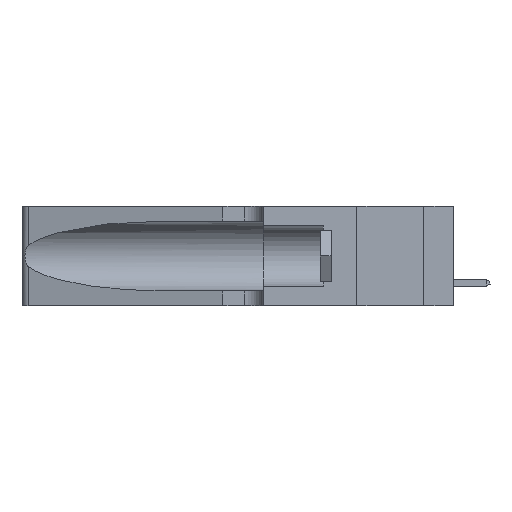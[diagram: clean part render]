
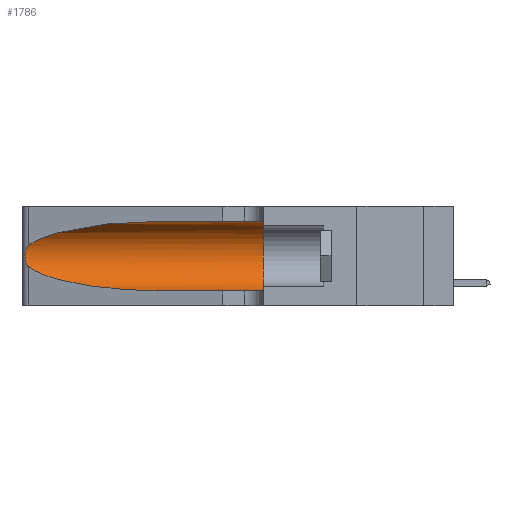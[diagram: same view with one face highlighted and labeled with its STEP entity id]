
A CAD part, left-side view. The second image highlights one B-rep face of the part: STEP entity #1786.
In plain terms, the highlighted cylindrical face has radius 3.308 mm (diameter 6.617 mm), a partial arc.
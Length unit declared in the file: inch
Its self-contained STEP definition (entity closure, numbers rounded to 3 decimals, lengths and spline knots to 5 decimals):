
#256 = FACE_OUTER_BOUND ( 'NONE', #6299, .T. ) ;
#331 = VERTEX_POINT ( 'NONE', #4029 ) ;
#347 = DIRECTION ( 'NONE',  ( 0., -1., 0. ) ) ;
#350 = VERTEX_POINT ( 'NONE', #19721 ) ;
#406 = VERTEX_POINT ( 'NONE', #17845 ) ;
#582 = DIRECTION ( 'NONE',  ( 0., 1., 0. ) ) ;
#608 = CARTESIAN_POINT ( 'NONE',  ( 0.26075, 1.23896, 0.19203 ) ) ;
#759 = VECTOR ( 'NONE', #5576, 39.37008 ) ;
#1049 = CARTESIAN_POINT ( 'NONE',  ( 0.1305, 0.72297, 0.05475 ) ) ;
#1786 = ADVANCED_FACE ( 'NONE', ( #256 ), #2389, .F. ) ;
#2276 = CARTESIAN_POINT ( 'NONE',  ( 0.18966, 0.96281, 0.31525 ) ) ;
#2389 = CYLINDRICAL_SURFACE ( 'NONE', #10808, 0.13025 ) ;
#2466 = AXIS2_PLACEMENT_3D ( 'NONE', #17288, #582, #11301 ) ;
#2964 = ORIENTED_EDGE ( 'NONE', *, *, #7996, .T. ) ;
#3274 = CARTESIAN_POINT ( 'NONE',  ( 0.1305, 1.61858, 0.185 ) ) ;
#4029 = CARTESIAN_POINT ( 'NONE',  ( 0.1305, 0.35, 0.31525 ) ) ;
#4107 = CARTESIAN_POINT ( 'NONE',  ( 0.25487, 1.22718, 0.22369 ) ) ;
#4141 = CARTESIAN_POINT ( 'NONE',  ( 0.25487, 1.22718, 0.22369 ) ) ;
#5185 = CARTESIAN_POINT ( 'NONE',  ( 0.25854, 1.2359, 0.20912 ) ) ;
#5260 = CARTESIAN_POINT ( 'NONE',  ( 0.1305, 0.72297, 0.31525 ) ) ;
#5356 = EDGE_CURVE ( 'NONE', #15737, #406, #15269, .T. ) ;
#5564 = CARTESIAN_POINT ( 'NONE',  ( 0.1305, 0.72297, 0.31525 ) ) ;
#5576 = DIRECTION ( 'NONE',  ( 0., -1., 0. ) ) ;
#6299 = EDGE_LOOP ( 'NONE', ( #13620, #9342, #15870, #2964, #8576, #19236 ) ) ;
#6657 = CARTESIAN_POINT ( 'NONE',  ( 0.25639, 1.23186, 0.15144 ) ) ;
#6722 = CARTESIAN_POINT ( 'NONE',  ( 0.25789, 1.23486, 0.15765 ) ) ;
#7068 = CARTESIAN_POINT ( 'NONE',  ( 0.18966, 0.96281, 0.05475 ) ) ;
#7996 = EDGE_CURVE ( 'NONE', #9312, #350, #9700, .T. ) ;
#8010 = DIRECTION ( 'NONE',  ( 0., 0., -1. ) ) ;
#8320 = CARTESIAN_POINT ( 'NONE',  ( 0.25787, 1.23484, 0.2124 ) ) ;
#8576 = ORIENTED_EDGE ( 'NONE', *, *, #9623, .F. ) ;
#8613 = CIRCLE ( 'NONE', #2466, 0.13025 ) ;
#8766 = CARTESIAN_POINT ( 'NONE',  ( 0.2373, 1.15595, 0.28018 ) ) ;
#9312 = VERTEX_POINT ( 'NONE', #11413 ) ;
#9342 = ORIENTED_EDGE ( 'NONE', *, *, #5356, .T. ) ;
#9623 = EDGE_CURVE ( 'NONE', #331, #350, #8613, .T. ) ;
#9700 = LINE ( 'NONE', #18607, #11139 ) ;
#9722 = CARTESIAN_POINT ( 'NONE',  ( 0.25639, 1.23184, 0.21858 ) ) ;
#10459 =( BOUNDED_CURVE ( )  B_SPLINE_CURVE ( 3, ( #5260, #2276, #8766, #4141 ),
 .UNSPECIFIED., .F., .F. ) 
 B_SPLINE_CURVE_WITH_KNOTS ( ( 4, 4 ),
 ( 1.5708, 2.84003 ),
 .UNSPECIFIED. ) 
 CURVE ( )  GEOMETRIC_REPRESENTATION_ITEM ( )  RATIONAL_B_SPLINE_CURVE ( ( 1., 0.87, 0.87, 1. ) ) 
 REPRESENTATION_ITEM ( '' )  );
#10808 = AXIS2_PLACEMENT_3D ( 'NONE', #3274, #347, #8010 ) ;
#11139 = VECTOR ( 'NONE', #13978, 39.37008 ) ;
#11252 = LINE ( 'NONE', #14785, #759 ) ;
#11258 = CARTESIAN_POINT ( 'NONE',  ( 0.25856, 1.23593, 0.16098 ) ) ;
#11301 = DIRECTION ( 'NONE',  ( 0., 0., 1. ) ) ;
#11413 = CARTESIAN_POINT ( 'NONE',  ( 0.1305, 0.72297, 0.05475 ) ) ;
#12943 =( BOUNDED_CURVE ( )  B_SPLINE_CURVE ( 3, ( #16429, #14669, #7068, #1049 ),
 .UNSPECIFIED., .F., .F. ) 
 B_SPLINE_CURVE_WITH_KNOTS ( ( 4, 4 ),
 ( 3.44316, 4.71239 ),
 .UNSPECIFIED. ) 
 CURVE ( )  GEOMETRIC_REPRESENTATION_ITEM ( )  RATIONAL_B_SPLINE_CURVE ( ( 1., 0.87, 0.87, 1. ) ) 
 REPRESENTATION_ITEM ( '' )  );
#13007 = CARTESIAN_POINT ( 'NONE',  ( 0.26075, 1.23896, 0.178 ) ) ;
#13487 = VERTEX_POINT ( 'NONE', #5564 ) ;
#13620 = ORIENTED_EDGE ( 'NONE', *, *, #17351, .T. ) ;
#13978 = DIRECTION ( 'NONE',  ( 0., -1., 0. ) ) ;
#14409 = CARTESIAN_POINT ( 'NONE',  ( 0.25555, 1.22994, 0.2215 ) ) ;
#14669 = CARTESIAN_POINT ( 'NONE',  ( 0.2373, 1.15595, 0.08982 ) ) ;
#14785 = CARTESIAN_POINT ( 'NONE',  ( 0.1305, 1.61858, 0.31525 ) ) ;
#15269 = B_SPLINE_CURVE_WITH_KNOTS ( 'NONE', 3,
 ( #18915, #14409, #9722, #8320, #5185, #15864, #608, #13007, #17441, #11258, #6722, #6657, #19107, #17367 ),
 .UNSPECIFIED., .F., .F.,
 ( 4, 2, 2, 2, 2, 2, 4 ),
 ( 0., 0.00027, 0.00053, 0.00107, 0.0016, 0.00187, 0.00214 ),
 .UNSPECIFIED. ) ;
#15737 = VERTEX_POINT ( 'NONE', #4107 ) ;
#15864 = CARTESIAN_POINT ( 'NONE',  ( 0.26018, 1.23835, 0.19895 ) ) ;
#15870 = ORIENTED_EDGE ( 'NONE', *, *, #18257, .T. ) ;
#16429 = CARTESIAN_POINT ( 'NONE',  ( 0.25487, 1.22718, 0.14631 ) ) ;
#17288 = CARTESIAN_POINT ( 'NONE',  ( 0.1305, 0.35, 0.185 ) ) ;
#17351 = EDGE_CURVE ( 'NONE', #13487, #15737, #10459, .T. ) ;
#17367 = CARTESIAN_POINT ( 'NONE',  ( 0.25487, 1.22718, 0.14631 ) ) ;
#17441 = CARTESIAN_POINT ( 'NONE',  ( 0.26017, 1.23833, 0.17102 ) ) ;
#17845 = CARTESIAN_POINT ( 'NONE',  ( 0.25487, 1.22718, 0.14631 ) ) ;
#18257 = EDGE_CURVE ( 'NONE', #406, #9312, #12943, .T. ) ;
#18305 = EDGE_CURVE ( 'NONE', #13487, #331, #11252, .T. ) ;
#18607 = CARTESIAN_POINT ( 'NONE',  ( 0.1305, 1.61858, 0.05475 ) ) ;
#18915 = CARTESIAN_POINT ( 'NONE',  ( 0.25487, 1.22718, 0.22369 ) ) ;
#19107 = CARTESIAN_POINT ( 'NONE',  ( 0.25555, 1.22993, 0.14849 ) ) ;
#19236 = ORIENTED_EDGE ( 'NONE', *, *, #18305, .F. ) ;
#19721 = CARTESIAN_POINT ( 'NONE',  ( 0.1305, 0.35, 0.05475 ) ) ;
